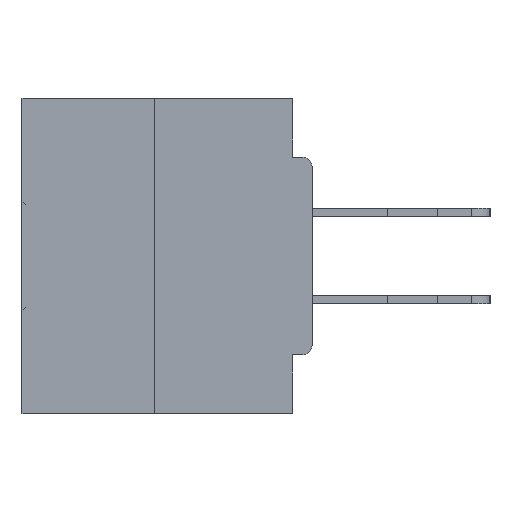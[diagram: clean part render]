
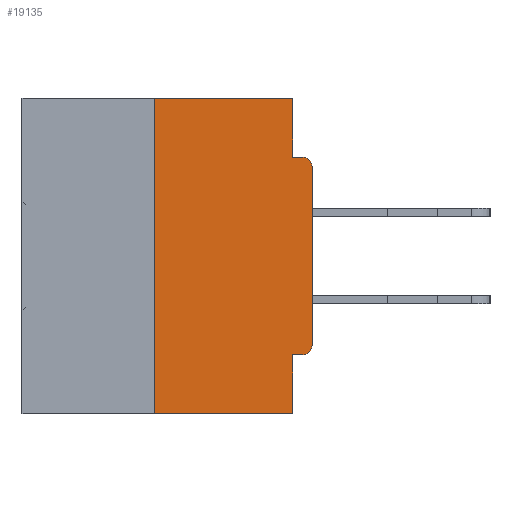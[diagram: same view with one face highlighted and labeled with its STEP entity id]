
A CAD part, left-side view. The second image highlights one B-rep face of the part: STEP entity #19135.
In plain terms, the highlighted planar face has unit normal (-1, 0, 0).
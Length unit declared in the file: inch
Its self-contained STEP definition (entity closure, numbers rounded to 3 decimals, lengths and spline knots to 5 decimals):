
#194 = EDGE_CURVE ( 'NONE', #2547, #34565, #16678, .T. ) ;
#1443 = EDGE_CURVE ( 'NONE', #34565, #4511, #2101, .T. ) ;
#1484 = DIRECTION ( 'NONE',  ( 0., 0., 1. ) ) ;
#1486 = DIRECTION ( 'NONE',  ( 0., -1., 0. ) ) ;
#1653 = FACE_OUTER_BOUND ( 'NONE', #12096, .T. ) ;
#2101 = LINE ( 'NONE', #4688, #32920 ) ;
#2547 = VERTEX_POINT ( 'NONE', #15701 ) ;
#3032 = VERTEX_POINT ( 'NONE', #10482 ) ;
#3660 = CARTESIAN_POINT ( 'NONE',  ( 0., 0.25, 0. ) ) ;
#4511 = VERTEX_POINT ( 'NONE', #27513 ) ;
#4638 = LINE ( 'NONE', #30046, #8304 ) ;
#4688 = CARTESIAN_POINT ( 'NONE',  ( 0., 0.031, -0.5 ) ) ;
#5097 = CARTESIAN_POINT ( 'NONE',  ( 0., 0., -0.0935 ) ) ;
#5577 = DIRECTION ( 'NONE',  ( 0., 0., -1. ) ) ;
#5880 = PLANE ( 'NONE',  #20849 ) ;
#6647 = CARTESIAN_POINT ( 'NONE',  ( 0., 0.031, -0.4065 ) ) ;
#6774 = DIRECTION ( 'NONE',  ( 0., -1., 0. ) ) ;
#6950 = VECTOR ( 'NONE', #8265, 39.37008 ) ;
#7004 = CARTESIAN_POINT ( 'NONE',  ( 0., 0.25, 0. ) ) ;
#7589 = VECTOR ( 'NONE', #22326, 39.37008 ) ;
#8029 = LINE ( 'NONE', #17882, #6950 ) ;
#8037 = CARTESIAN_POINT ( 'NONE',  ( 0., 0., -0.3915 ) ) ;
#8109 = EDGE_CURVE ( 'NONE', #2547, #17474, #14791, .T. ) ;
#8160 = CARTESIAN_POINT ( 'NONE',  ( 0., 0.015, -0.3915 ) ) ;
#8265 = DIRECTION ( 'NONE',  ( 0., 0., -1. ) ) ;
#8304 = VECTOR ( 'NONE', #23152, 39.37008 ) ;
#9305 = CARTESIAN_POINT ( 'NONE',  ( 0., 0.46, -0.5 ) ) ;
#9945 = EDGE_CURVE ( 'NONE', #24947, #12780, #34547, .T. ) ;
#10093 = EDGE_CURVE ( 'NONE', #40488, #21559, #38122, .T. ) ;
#10482 = CARTESIAN_POINT ( 'NONE',  ( 0., 0.25, -0.5 ) ) ;
#10501 = VECTOR ( 'NONE', #31207, 39.37008 ) ;
#12096 = EDGE_LOOP ( 'NONE', ( #25563, #14977, #19532, #19472, #40563, #36435, #31222, #39918, #39520, #19263 ) ) ;
#12113 = DIRECTION ( 'NONE',  ( 1., 0., 0. ) ) ;
#12780 = VERTEX_POINT ( 'NONE', #37105 ) ;
#13301 = EDGE_CURVE ( 'NONE', #41910, #12780, #26022, .T. ) ;
#13930 = CARTESIAN_POINT ( 'NONE',  ( 0., 0.031, -0.0935 ) ) ;
#14791 = CIRCLE ( 'NONE', #17774, 0.015 ) ;
#14977 = ORIENTED_EDGE ( 'NONE', *, *, #38021, .F. ) ;
#15354 = EDGE_CURVE ( 'NONE', #21559, #41910, #8029, .T. ) ;
#15701 = CARTESIAN_POINT ( 'NONE',  ( 0., 0.015, -0.4065 ) ) ;
#16678 = LINE ( 'NONE', #30931, #10501 ) ;
#17474 = VERTEX_POINT ( 'NONE', #8037 ) ;
#17774 = AXIS2_PLACEMENT_3D ( 'NONE', #8160, #36951, #21057 ) ;
#17882 = CARTESIAN_POINT ( 'NONE',  ( 0., 0.031, 0. ) ) ;
#18514 = DIRECTION ( 'NONE',  ( -1., 0., 0. ) ) ;
#19135 = ADVANCED_FACE ( 'NONE', ( #1653 ), #5880, .F. ) ;
#19263 = ORIENTED_EDGE ( 'NONE', *, *, #15354, .F. ) ;
#19472 = ORIENTED_EDGE ( 'NONE', *, *, #1443, .F. ) ;
#19532 = ORIENTED_EDGE ( 'NONE', *, *, #41698, .T. ) ;
#19622 = VECTOR ( 'NONE', #6774, 39.37008 ) ;
#20820 = CARTESIAN_POINT ( 'NONE',  ( 0., 0.031, 0. ) ) ;
#20849 = AXIS2_PLACEMENT_3D ( 'NONE', #21968, #12113, #35299 ) ;
#21057 = DIRECTION ( 'NONE',  ( 0., 0., -1. ) ) ;
#21559 = VERTEX_POINT ( 'NONE', #20820 ) ;
#21968 = CARTESIAN_POINT ( 'NONE',  ( 0., 0.46, 0. ) ) ;
#22326 = DIRECTION ( 'NONE',  ( 0., -1., 0. ) ) ;
#23152 = DIRECTION ( 'NONE',  ( 0., 0., 1. ) ) ;
#23523 = CARTESIAN_POINT ( 'NONE',  ( 0., 0.46, 0. ) ) ;
#24947 = VERTEX_POINT ( 'NONE', #38740 ) ;
#25563 = ORIENTED_EDGE ( 'NONE', *, *, #10093, .F. ) ;
#26022 = LINE ( 'NONE', #5097, #39922 ) ;
#27513 = CARTESIAN_POINT ( 'NONE',  ( 0., 0.031, -0.5 ) ) ;
#29104 = LINE ( 'NONE', #9305, #7589 ) ;
#30046 = CARTESIAN_POINT ( 'NONE',  ( 0., 0., 0. ) ) ;
#30931 = CARTESIAN_POINT ( 'NONE',  ( 0., 0., -0.4065 ) ) ;
#31207 = DIRECTION ( 'NONE',  ( 0., 1., 0. ) ) ;
#31222 = ORIENTED_EDGE ( 'NONE', *, *, #36268, .T. ) ;
#32522 = LINE ( 'NONE', #3660, #35621 ) ;
#32920 = VECTOR ( 'NONE', #34397, 39.37008 ) ;
#34397 = DIRECTION ( 'NONE',  ( 0., 0., -1. ) ) ;
#34547 = CIRCLE ( 'NONE', #38167, 0.015 ) ;
#34565 = VERTEX_POINT ( 'NONE', #6647 ) ;
#35299 = DIRECTION ( 'NONE',  ( 0., 0., -1. ) ) ;
#35621 = VECTOR ( 'NONE', #1484, 39.37008 ) ;
#36268 = EDGE_CURVE ( 'NONE', #17474, #24947, #4638, .T. ) ;
#36435 = ORIENTED_EDGE ( 'NONE', *, *, #8109, .T. ) ;
#36951 = DIRECTION ( 'NONE',  ( -1., 0., 0. ) ) ;
#37105 = CARTESIAN_POINT ( 'NONE',  ( 0., 0.015, -0.0935 ) ) ;
#38021 = EDGE_CURVE ( 'NONE', #3032, #40488, #32522, .T. ) ;
#38122 = LINE ( 'NONE', #23523, #19622 ) ;
#38167 = AXIS2_PLACEMENT_3D ( 'NONE', #41180, #18514, #5577 ) ;
#38740 = CARTESIAN_POINT ( 'NONE',  ( 0., 0., -0.1085 ) ) ;
#39520 = ORIENTED_EDGE ( 'NONE', *, *, #13301, .F. ) ;
#39918 = ORIENTED_EDGE ( 'NONE', *, *, #9945, .T. ) ;
#39922 = VECTOR ( 'NONE', #1486, 39.37008 ) ;
#40488 = VERTEX_POINT ( 'NONE', #7004 ) ;
#40563 = ORIENTED_EDGE ( 'NONE', *, *, #194, .F. ) ;
#41180 = CARTESIAN_POINT ( 'NONE',  ( 0., 0.015, -0.1085 ) ) ;
#41698 = EDGE_CURVE ( 'NONE', #3032, #4511, #29104, .T. ) ;
#41910 = VERTEX_POINT ( 'NONE', #13930 ) ;
